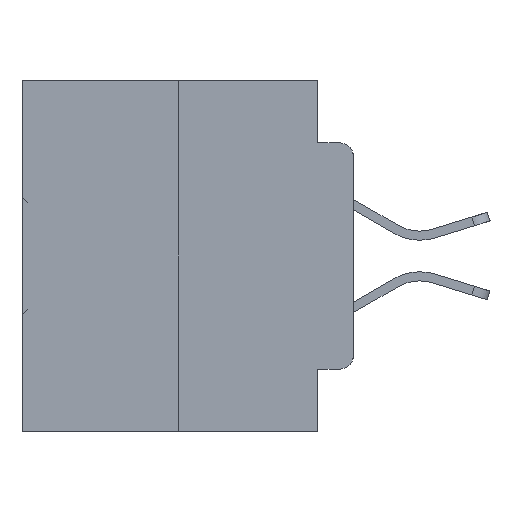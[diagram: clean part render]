
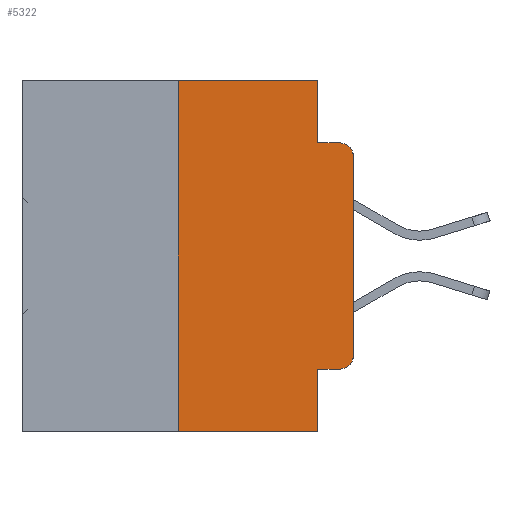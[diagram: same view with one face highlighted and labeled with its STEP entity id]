
A CAD part, left-side view. The second image highlights one B-rep face of the part: STEP entity #5322.
In plain terms, the highlighted planar face has unit normal (-1, 0, 0).
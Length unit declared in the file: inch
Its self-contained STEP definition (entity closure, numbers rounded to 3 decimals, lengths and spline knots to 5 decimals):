
#285 = ORIENTED_EDGE ( 'NONE', *, *, #6033, .T. ) ;
#781 = CARTESIAN_POINT ( 'NONE',  ( 0., 0.25, 0. ) ) ;
#1503 = DIRECTION ( 'NONE',  ( 0., 0., -1. ) ) ;
#2530 = DIRECTION ( 'NONE',  ( 1., 0., 0. ) ) ;
#3033 = PLANE ( 'NONE',  #6841 ) ;
#3303 = DIRECTION ( 'NONE',  ( 0., -1., 0. ) ) ;
#4275 = EDGE_CURVE ( 'NONE', #17808, #6219, #20000, .T. ) ;
#4433 = ORIENTED_EDGE ( 'NONE', *, *, #14237, .T. ) ;
#5322 = ADVANCED_FACE ( 'NONE', ( #14011 ), #3033, .F. ) ;
#5804 = ORIENTED_EDGE ( 'NONE', *, *, #32653, .T. ) ;
#6028 = CARTESIAN_POINT ( 'NONE',  ( 0., 0.473, 0. ) ) ;
#6033 = EDGE_CURVE ( 'NONE', #13590, #11967, #32810, .T. ) ;
#6219 = VERTEX_POINT ( 'NONE', #11170 ) ;
#6325 = VECTOR ( 'NONE', #9381, 39.37008 ) ;
#6604 = ORIENTED_EDGE ( 'NONE', *, *, #4275, .F. ) ;
#6649 = CARTESIAN_POINT ( 'NONE',  ( 0., 0., 0. ) ) ;
#6841 = AXIS2_PLACEMENT_3D ( 'NONE', #9312, #2530, #27519 ) ;
#7104 = LINE ( 'NONE', #33336, #27491 ) ;
#7127 = CARTESIAN_POINT ( 'NONE',  ( 0., 0.473, -0.5 ) ) ;
#7833 = DIRECTION ( 'NONE',  ( -1., 0., 0. ) ) ;
#8517 = VECTOR ( 'NONE', #21833, 39.37008 ) ;
#8622 = DIRECTION ( 'NONE',  ( -1., 0., 0. ) ) ;
#9033 = CARTESIAN_POINT ( 'NONE',  ( 0., 0.051, -0.4115 ) ) ;
#9207 = DIRECTION ( 'NONE',  ( 0., 0., -1. ) ) ;
#9312 = CARTESIAN_POINT ( 'NONE',  ( 0., 0.473, 0. ) ) ;
#9381 = DIRECTION ( 'NONE',  ( 0., 0., 1. ) ) ;
#9527 = CARTESIAN_POINT ( 'NONE',  ( 0., 0.051, 0. ) ) ;
#11114 = VERTEX_POINT ( 'NONE', #18083 ) ;
#11170 = CARTESIAN_POINT ( 'NONE',  ( 0., 0.051, -0.0885 ) ) ;
#11300 = CARTESIAN_POINT ( 'NONE',  ( 0., 0.02, -0.4115 ) ) ;
#11311 = CARTESIAN_POINT ( 'NONE',  ( 0., 0.051, -0.0885 ) ) ;
#11544 = CARTESIAN_POINT ( 'NONE',  ( 0., 0.051, -0.4115 ) ) ;
#11967 = VERTEX_POINT ( 'NONE', #20294 ) ;
#13187 = CIRCLE ( 'NONE', #23843, 0.02 ) ;
#13590 = VERTEX_POINT ( 'NONE', #11300 ) ;
#13825 = VECTOR ( 'NONE', #30111, 39.37008 ) ;
#14011 = FACE_OUTER_BOUND ( 'NONE', #34144, .T. ) ;
#14237 = EDGE_CURVE ( 'NONE', #11114, #25263, #13187, .T. ) ;
#14260 = ORIENTED_EDGE ( 'NONE', *, *, #27683, .T. ) ;
#14666 = VECTOR ( 'NONE', #9207, 39.37008 ) ;
#14882 = EDGE_CURVE ( 'NONE', #11967, #11114, #27548, .T. ) ;
#15283 = VECTOR ( 'NONE', #25762, 39.37008 ) ;
#15475 = ORIENTED_EDGE ( 'NONE', *, *, #23920, .F. ) ;
#15866 = ORIENTED_EDGE ( 'NONE', *, *, #21287, .F. ) ;
#15898 = ORIENTED_EDGE ( 'NONE', *, *, #31565, .F. ) ;
#16850 = EDGE_CURVE ( 'NONE', #27542, #26865, #30272, .T. ) ;
#17056 = ORIENTED_EDGE ( 'NONE', *, *, #14882, .T. ) ;
#17144 = VECTOR ( 'NONE', #3303, 39.37008 ) ;
#17808 = VERTEX_POINT ( 'NONE', #33232 ) ;
#17917 = CARTESIAN_POINT ( 'NONE',  ( 0., 0.25, 0. ) ) ;
#17973 = LINE ( 'NONE', #6028, #17144 ) ;
#18083 = CARTESIAN_POINT ( 'NONE',  ( 0., 0., -0.1085 ) ) ;
#20000 = LINE ( 'NONE', #9527, #14666 ) ;
#20294 = CARTESIAN_POINT ( 'NONE',  ( 0., 0., -0.3915 ) ) ;
#20814 = LINE ( 'NONE', #11544, #13825 ) ;
#21287 = EDGE_CURVE ( 'NONE', #6219, #25263, #30483, .T. ) ;
#21447 = LINE ( 'NONE', #7127, #15283 ) ;
#21833 = DIRECTION ( 'NONE',  ( 0., -1., 0. ) ) ;
#22739 = CARTESIAN_POINT ( 'NONE',  ( 0., 0.02, -0.0885 ) ) ;
#23072 = DIRECTION ( 'NONE',  ( 0., 0., -1. ) ) ;
#23357 = VERTEX_POINT ( 'NONE', #30323 ) ;
#23811 = CARTESIAN_POINT ( 'NONE',  ( 0., 0.02, -0.3915 ) ) ;
#23843 = AXIS2_PLACEMENT_3D ( 'NONE', #24570, #8622, #23072 ) ;
#23920 = EDGE_CURVE ( 'NONE', #26865, #17808, #17973, .T. ) ;
#24570 = CARTESIAN_POINT ( 'NONE',  ( 0., 0.02, -0.1085 ) ) ;
#25189 = AXIS2_PLACEMENT_3D ( 'NONE', #23811, #7833, #26441 ) ;
#25263 = VERTEX_POINT ( 'NONE', #22739 ) ;
#25762 = DIRECTION ( 'NONE',  ( 0., -1., 0. ) ) ;
#25799 = ORIENTED_EDGE ( 'NONE', *, *, #16850, .F. ) ;
#26441 = DIRECTION ( 'NONE',  ( 0., 0., -1. ) ) ;
#26865 = VERTEX_POINT ( 'NONE', #781 ) ;
#27491 = VECTOR ( 'NONE', #1503, 39.37008 ) ;
#27502 = VERTEX_POINT ( 'NONE', #9033 ) ;
#27519 = DIRECTION ( 'NONE',  ( 0., 0., -1. ) ) ;
#27542 = VERTEX_POINT ( 'NONE', #30446 ) ;
#27548 = LINE ( 'NONE', #6649, #6325 ) ;
#27683 = EDGE_CURVE ( 'NONE', #27542, #23357, #21447, .T. ) ;
#29463 = VECTOR ( 'NONE', #31000, 39.37008 ) ;
#30111 = DIRECTION ( 'NONE',  ( 0., -1., 0. ) ) ;
#30272 = LINE ( 'NONE', #17917, #29463 ) ;
#30323 = CARTESIAN_POINT ( 'NONE',  ( 0., 0.051, -0.5 ) ) ;
#30446 = CARTESIAN_POINT ( 'NONE',  ( 0., 0.25, -0.5 ) ) ;
#30483 = LINE ( 'NONE', #11311, #8517 ) ;
#31000 = DIRECTION ( 'NONE',  ( 0., 0., 1. ) ) ;
#31565 = EDGE_CURVE ( 'NONE', #27502, #23357, #7104, .T. ) ;
#32653 = EDGE_CURVE ( 'NONE', #27502, #13590, #20814, .T. ) ;
#32810 = CIRCLE ( 'NONE', #25189, 0.02 ) ;
#33232 = CARTESIAN_POINT ( 'NONE',  ( 0., 0.051, 0. ) ) ;
#33336 = CARTESIAN_POINT ( 'NONE',  ( 0., 0.051, 0. ) ) ;
#34144 = EDGE_LOOP ( 'NONE', ( #17056, #4433, #15866, #6604, #15475, #25799, #14260, #15898, #5804, #285 ) ) ;
